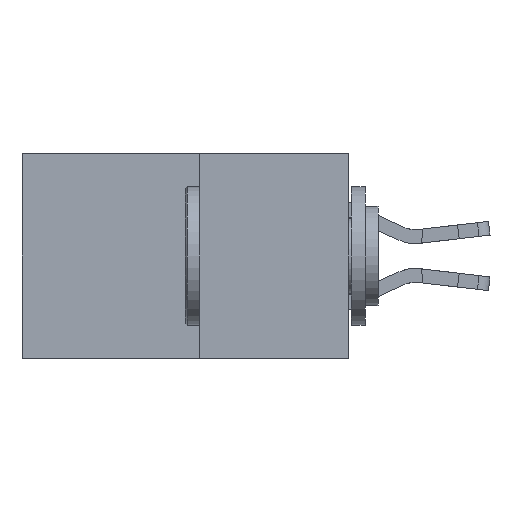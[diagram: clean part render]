
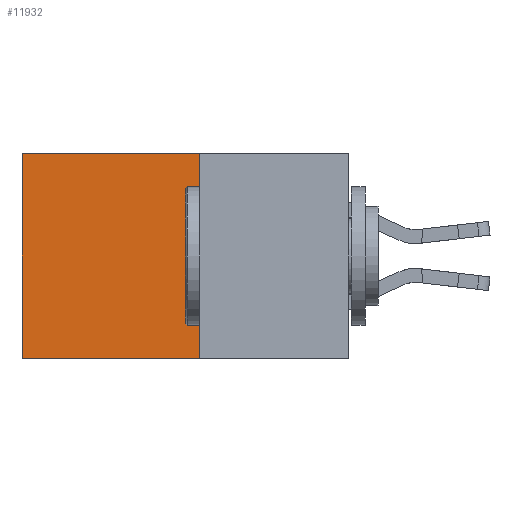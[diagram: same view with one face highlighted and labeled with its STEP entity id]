
A CAD part, left-side view. The second image highlights one B-rep face of the part: STEP entity #11932.
In plain terms, the highlighted planar face has unit normal (-1, 0, 0).
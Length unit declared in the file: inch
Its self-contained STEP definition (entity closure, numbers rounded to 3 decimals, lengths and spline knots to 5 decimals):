
#276 = EDGE_CURVE ( 'NONE', #13967, #2820, #5863, .T. ) ;
#364 = ORIENTED_EDGE ( 'NONE', *, *, #6456, .T. ) ;
#2296 = FACE_OUTER_BOUND ( 'NONE', #2638, .T. ) ;
#2638 = EDGE_LOOP ( 'NONE', ( #9384, #9703, #4310, #364 ) ) ;
#2820 = VERTEX_POINT ( 'NONE', #6311 ) ;
#3896 = CARTESIAN_POINT ( 'NONE',  ( 0.277, 0.27, -0.37 ) ) ;
#4057 = VECTOR ( 'NONE', #7040, 39.37008 ) ;
#4310 = ORIENTED_EDGE ( 'NONE', *, *, #7854, .F. ) ;
#5863 = LINE ( 'NONE', #10748, #10574 ) ;
#6134 = DIRECTION ( 'NONE',  ( 1., 0., 0. ) ) ;
#6309 = CARTESIAN_POINT ( 'NONE',  ( 0.277, 0.27, -0.37 ) ) ;
#6311 = CARTESIAN_POINT ( 'NONE',  ( 0.277, 0.59, -0.37 ) ) ;
#6456 = EDGE_CURVE ( 'NONE', #13121, #13967, #7279, .T. ) ;
#7040 = DIRECTION ( 'NONE',  ( 0., 1., 0. ) ) ;
#7180 = CARTESIAN_POINT ( 'NONE',  ( 0.277, 0.27, 0. ) ) ;
#7279 = LINE ( 'NONE', #7180, #4057 ) ;
#7854 = EDGE_CURVE ( 'NONE', #13121, #10710, #9784, .T. ) ;
#8197 = CARTESIAN_POINT ( 'NONE',  ( 0.277, 0.27, 0. ) ) ;
#9274 = LINE ( 'NONE', #6309, #11417 ) ;
#9384 = ORIENTED_EDGE ( 'NONE', *, *, #276, .T. ) ;
#9429 = CARTESIAN_POINT ( 'NONE',  ( 0.277, 0.27, -0.37 ) ) ;
#9453 = VECTOR ( 'NONE', #9785, 39.37008 ) ;
#9586 = DIRECTION ( 'NONE',  ( 0., 1., 0. ) ) ;
#9703 = ORIENTED_EDGE ( 'NONE', *, *, #12059, .F. ) ;
#9784 = LINE ( 'NONE', #10839, #9453 ) ;
#9785 = DIRECTION ( 'NONE',  ( 0., 0., -1. ) ) ;
#10574 = VECTOR ( 'NONE', #13404, 39.37008 ) ;
#10710 = VERTEX_POINT ( 'NONE', #9429 ) ;
#10748 = CARTESIAN_POINT ( 'NONE',  ( 0.277, 0.59, -0.37 ) ) ;
#10839 = CARTESIAN_POINT ( 'NONE',  ( 0.277, 0.27, -0.37 ) ) ;
#11235 = AXIS2_PLACEMENT_3D ( 'NONE', #3896, #6134, #13505 ) ;
#11417 = VECTOR ( 'NONE', #9586, 39.37008 ) ;
#11932 = ADVANCED_FACE ( 'NONE', ( #2296 ), #12495, .F. ) ;
#12059 = EDGE_CURVE ( 'NONE', #10710, #2820, #9274, .T. ) ;
#12068 = CARTESIAN_POINT ( 'NONE',  ( 0.277, 0.59, 0. ) ) ;
#12495 = PLANE ( 'NONE',  #11235 ) ;
#13121 = VERTEX_POINT ( 'NONE', #8197 ) ;
#13404 = DIRECTION ( 'NONE',  ( 0., 0., -1. ) ) ;
#13505 = DIRECTION ( 'NONE',  ( 0., 0., -1. ) ) ;
#13967 = VERTEX_POINT ( 'NONE', #12068 ) ;
